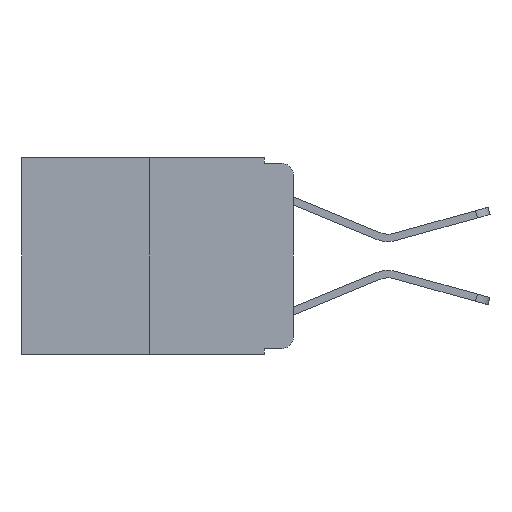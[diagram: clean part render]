
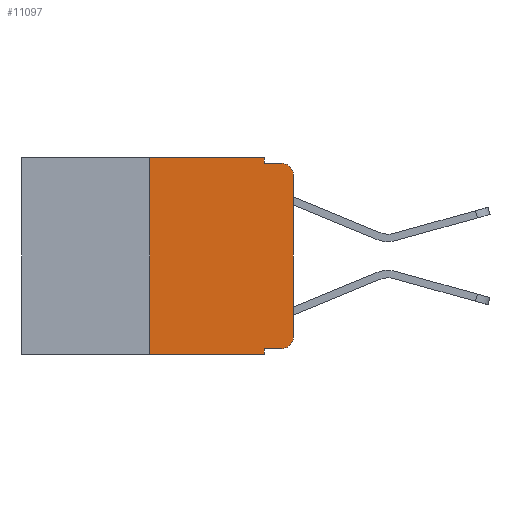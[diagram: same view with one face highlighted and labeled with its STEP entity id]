
A CAD part, left-side view. The second image highlights one B-rep face of the part: STEP entity #11097.
In plain terms, the highlighted planar face has unit normal (-1, 0, 0).
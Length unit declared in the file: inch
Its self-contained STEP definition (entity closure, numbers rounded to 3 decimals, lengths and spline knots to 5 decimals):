
#103 = VECTOR ( 'NONE', #1211, 39.37008 ) ;
#139 = VECTOR ( 'NONE', #8634, 39.37008 ) ;
#237 = DIRECTION ( 'NONE',  ( 0., 0., -1. ) ) ;
#261 = CIRCLE ( 'NONE', #1518, 0.02 ) ;
#474 = ORIENTED_EDGE ( 'NONE', *, *, #8697, .T. ) ;
#1002 = VERTEX_POINT ( 'NONE', #11543 ) ;
#1020 = DIRECTION ( 'NONE',  ( 0., -1., 0. ) ) ;
#1040 = EDGE_CURVE ( 'NONE', #10008, #6176, #261, .T. ) ;
#1211 = DIRECTION ( 'NONE',  ( 0., 0., 1. ) ) ;
#1253 = CARTESIAN_POINT ( 'NONE',  ( 0., 0.473, -0.343 ) ) ;
#1512 = ORIENTED_EDGE ( 'NONE', *, *, #9838, .F. ) ;
#1518 = AXIS2_PLACEMENT_3D ( 'NONE', #12587, #5693, #11602 ) ;
#1704 = ORIENTED_EDGE ( 'NONE', *, *, #2888, .T. ) ;
#1719 = VERTEX_POINT ( 'NONE', #10111 ) ;
#1924 = EDGE_LOOP ( 'NONE', ( #12064, #5838, #8082, #10847, #5603, #7997, #474, #1512, #1704, #9620 ) ) ;
#1970 = FACE_OUTER_BOUND ( 'NONE', #1924, .T. ) ;
#2168 = PLANE ( 'NONE',  #5825 ) ;
#2186 = CARTESIAN_POINT ( 'NONE',  ( 0., 0.051, -0.01 ) ) ;
#2219 = LINE ( 'NONE', #8266, #2450 ) ;
#2450 = VECTOR ( 'NONE', #237, 39.37008 ) ;
#2817 = VERTEX_POINT ( 'NONE', #3767 ) ;
#2888 = EDGE_CURVE ( 'NONE', #2817, #3221, #3828, .T. ) ;
#3147 = EDGE_CURVE ( 'NONE', #8492, #5927, #8641, .T. ) ;
#3160 = DIRECTION ( 'NONE',  ( 0., -1., 0. ) ) ;
#3178 = LINE ( 'NONE', #5074, #103 ) ;
#3221 = VERTEX_POINT ( 'NONE', #6408 ) ;
#3424 = VECTOR ( 'NONE', #7531, 39.37008 ) ;
#3767 = CARTESIAN_POINT ( 'NONE',  ( 0., 0.051, -0.333 ) ) ;
#3828 = LINE ( 'NONE', #12940, #6701 ) ;
#3902 = LINE ( 'NONE', #5350, #5212 ) ;
#4114 = AXIS2_PLACEMENT_3D ( 'NONE', #11933, #9009, #6972 ) ;
#4277 = EDGE_CURVE ( 'NONE', #11995, #6176, #3902, .T. ) ;
#4370 = CARTESIAN_POINT ( 'NONE',  ( 0., 0.051, 0. ) ) ;
#5074 = CARTESIAN_POINT ( 'NONE',  ( 0., 0., 0. ) ) ;
#5193 = LINE ( 'NONE', #1253, #6216 ) ;
#5212 = VECTOR ( 'NONE', #8199, 39.37008 ) ;
#5350 = CARTESIAN_POINT ( 'NONE',  ( 0., 0.051, -0.01 ) ) ;
#5603 = ORIENTED_EDGE ( 'NONE', *, *, #3147, .F. ) ;
#5693 = DIRECTION ( 'NONE',  ( -1., 0., 0. ) ) ;
#5748 = VECTOR ( 'NONE', #6481, 39.37008 ) ;
#5825 = AXIS2_PLACEMENT_3D ( 'NONE', #12073, #10197, #9011 ) ;
#5838 = ORIENTED_EDGE ( 'NONE', *, *, #1040, .T. ) ;
#5927 = VERTEX_POINT ( 'NONE', #10287 ) ;
#6176 = VERTEX_POINT ( 'NONE', #11220 ) ;
#6216 = VECTOR ( 'NONE', #3160, 39.37008 ) ;
#6408 = CARTESIAN_POINT ( 'NONE',  ( 0., 0.02, -0.333 ) ) ;
#6481 = DIRECTION ( 'NONE',  ( 0., 0., -1. ) ) ;
#6594 = LINE ( 'NONE', #9438, #139 ) ;
#6607 = LINE ( 'NONE', #4370, #5748 ) ;
#6701 = VECTOR ( 'NONE', #1020, 39.37008 ) ;
#6711 = EDGE_CURVE ( 'NONE', #5927, #11995, #6607, .T. ) ;
#6972 = DIRECTION ( 'NONE',  ( 0., 0., -1. ) ) ;
#7052 = EDGE_CURVE ( 'NONE', #12169, #10008, #3178, .T. ) ;
#7412 = CARTESIAN_POINT ( 'NONE',  ( 0., 0., -0.03 ) ) ;
#7531 = DIRECTION ( 'NONE',  ( 0., -1., 0. ) ) ;
#7997 = ORIENTED_EDGE ( 'NONE', *, *, #10409, .F. ) ;
#8030 = EDGE_CURVE ( 'NONE', #3221, #12169, #12684, .T. ) ;
#8082 = ORIENTED_EDGE ( 'NONE', *, *, #4277, .F. ) ;
#8199 = DIRECTION ( 'NONE',  ( 0., -1., 0. ) ) ;
#8266 = CARTESIAN_POINT ( 'NONE',  ( 0., 0.051, 0. ) ) ;
#8492 = VERTEX_POINT ( 'NONE', #12233 ) ;
#8634 = DIRECTION ( 'NONE',  ( 0., 0., 1. ) ) ;
#8641 = LINE ( 'NONE', #9643, #3424 ) ;
#8697 = EDGE_CURVE ( 'NONE', #1719, #1002, #5193, .T. ) ;
#9009 = DIRECTION ( 'NONE',  ( -1., 0., 0. ) ) ;
#9011 = DIRECTION ( 'NONE',  ( 0., 0., -1. ) ) ;
#9438 = CARTESIAN_POINT ( 'NONE',  ( 0., 0.25, 0. ) ) ;
#9620 = ORIENTED_EDGE ( 'NONE', *, *, #8030, .T. ) ;
#9643 = CARTESIAN_POINT ( 'NONE',  ( 0., 0.473, 0. ) ) ;
#9838 = EDGE_CURVE ( 'NONE', #2817, #1002, #2219, .T. ) ;
#10008 = VERTEX_POINT ( 'NONE', #7412 ) ;
#10111 = CARTESIAN_POINT ( 'NONE',  ( 0., 0.25, -0.343 ) ) ;
#10197 = DIRECTION ( 'NONE',  ( 1., 0., 0. ) ) ;
#10287 = CARTESIAN_POINT ( 'NONE',  ( 0., 0.051, 0. ) ) ;
#10409 = EDGE_CURVE ( 'NONE', #1719, #8492, #6594, .T. ) ;
#10847 = ORIENTED_EDGE ( 'NONE', *, *, #6711, .F. ) ;
#11097 = ADVANCED_FACE ( 'NONE', ( #1970 ), #2168, .F. ) ;
#11220 = CARTESIAN_POINT ( 'NONE',  ( 0., 0.02, -0.01 ) ) ;
#11543 = CARTESIAN_POINT ( 'NONE',  ( 0., 0.051, -0.343 ) ) ;
#11554 = CARTESIAN_POINT ( 'NONE',  ( 0., 0., -0.313 ) ) ;
#11602 = DIRECTION ( 'NONE',  ( 0., 0., -1. ) ) ;
#11933 = CARTESIAN_POINT ( 'NONE',  ( 0., 0.02, -0.313 ) ) ;
#11995 = VERTEX_POINT ( 'NONE', #2186 ) ;
#12064 = ORIENTED_EDGE ( 'NONE', *, *, #7052, .T. ) ;
#12073 = CARTESIAN_POINT ( 'NONE',  ( 0., 0.473, 0. ) ) ;
#12169 = VERTEX_POINT ( 'NONE', #11554 ) ;
#12233 = CARTESIAN_POINT ( 'NONE',  ( 0., 0.25, 0. ) ) ;
#12587 = CARTESIAN_POINT ( 'NONE',  ( 0., 0.02, -0.03 ) ) ;
#12684 = CIRCLE ( 'NONE', #4114, 0.02 ) ;
#12940 = CARTESIAN_POINT ( 'NONE',  ( 0., 0.051, -0.333 ) ) ;
